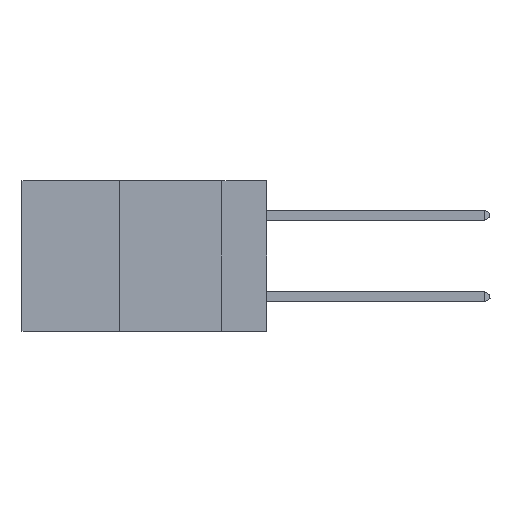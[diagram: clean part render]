
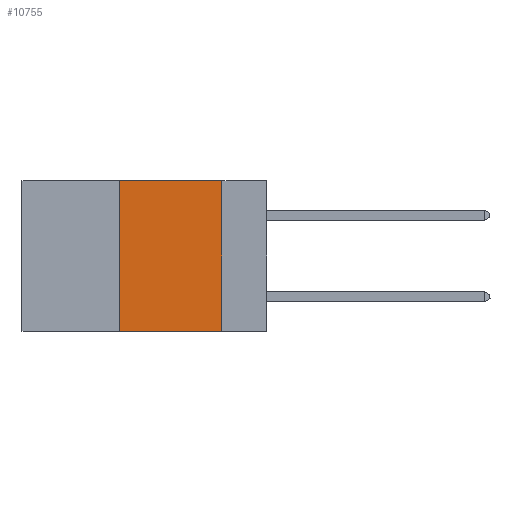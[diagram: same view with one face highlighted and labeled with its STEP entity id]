
A CAD part, left-side view. The second image highlights one B-rep face of the part: STEP entity #10755.
In plain terms, the highlighted planar face has unit normal (-1, 0, 0).
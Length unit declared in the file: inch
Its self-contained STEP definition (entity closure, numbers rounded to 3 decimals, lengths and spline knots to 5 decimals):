
#100 = VECTOR ( 'NONE', #4297, 39.37008 ) ;
#141 = CARTESIAN_POINT ( 'NONE',  ( 0., 0.36, 0. ) ) ;
#1571 = DIRECTION ( 'NONE',  ( 0., -1., 0. ) ) ;
#1594 = CARTESIAN_POINT ( 'NONE',  ( 0., 0.36, -0.37 ) ) ;
#1929 = DIRECTION ( 'NONE',  ( 0., 0., -1. ) ) ;
#2624 = AXIS2_PLACEMENT_3D ( 'NONE', #13362, #8203, #1929 ) ;
#2697 = EDGE_CURVE ( 'NONE', #10489, #4761, #13153, .T. ) ;
#2762 = VECTOR ( 'NONE', #5553, 39.37008 ) ;
#3298 = VERTEX_POINT ( 'NONE', #12029 ) ;
#3461 = EDGE_CURVE ( 'NONE', #10489, #3298, #8450, .T. ) ;
#3655 = CARTESIAN_POINT ( 'NONE',  ( 0., 0.6, -0.37 ) ) ;
#3928 = PLANE ( 'NONE',  #2624 ) ;
#4297 = DIRECTION ( 'NONE',  ( 0., 0., 1. ) ) ;
#4761 = VERTEX_POINT ( 'NONE', #12769 ) ;
#4959 = ORIENTED_EDGE ( 'NONE', *, *, #2697, .T. ) ;
#5553 = DIRECTION ( 'NONE',  ( 0., 0., -1. ) ) ;
#5690 = VERTEX_POINT ( 'NONE', #7504 ) ;
#6418 = EDGE_CURVE ( 'NONE', #5690, #4761, #8321, .T. ) ;
#7504 = CARTESIAN_POINT ( 'NONE',  ( 0., 0.11, 0. ) ) ;
#8203 = DIRECTION ( 'NONE',  ( 1., 0., 0. ) ) ;
#8321 = LINE ( 'NONE', #12794, #2762 ) ;
#8450 = LINE ( 'NONE', #141, #100 ) ;
#8602 = ORIENTED_EDGE ( 'NONE', *, *, #3461, .F. ) ;
#9890 = ORIENTED_EDGE ( 'NONE', *, *, #6418, .F. ) ;
#9912 = VECTOR ( 'NONE', #12918, 39.37008 ) ;
#10265 = FACE_OUTER_BOUND ( 'NONE', #13060, .T. ) ;
#10389 = ORIENTED_EDGE ( 'NONE', *, *, #12969, .F. ) ;
#10489 = VERTEX_POINT ( 'NONE', #1594 ) ;
#10755 = ADVANCED_FACE ( 'NONE', ( #10265 ), #3928, .F. ) ;
#11425 = VECTOR ( 'NONE', #1571, 39.37008 ) ;
#12029 = CARTESIAN_POINT ( 'NONE',  ( 0., 0.36, 0. ) ) ;
#12769 = CARTESIAN_POINT ( 'NONE',  ( 0., 0.11, -0.37 ) ) ;
#12794 = CARTESIAN_POINT ( 'NONE',  ( 0., 0.11, 0. ) ) ;
#12918 = DIRECTION ( 'NONE',  ( 0., -1., 0. ) ) ;
#12933 = CARTESIAN_POINT ( 'NONE',  ( 0., 0.6, 0. ) ) ;
#12969 = EDGE_CURVE ( 'NONE', #3298, #5690, #13240, .T. ) ;
#13060 = EDGE_LOOP ( 'NONE', ( #9890, #10389, #8602, #4959 ) ) ;
#13153 = LINE ( 'NONE', #3655, #9912 ) ;
#13240 = LINE ( 'NONE', #12933, #11425 ) ;
#13362 = CARTESIAN_POINT ( 'NONE',  ( 0., 0.6, 0. ) ) ;
